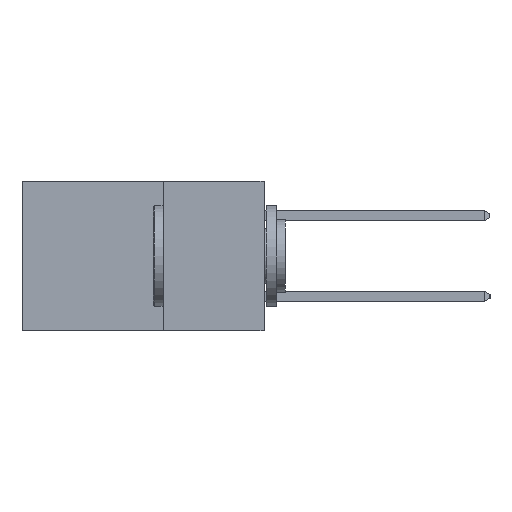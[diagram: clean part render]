
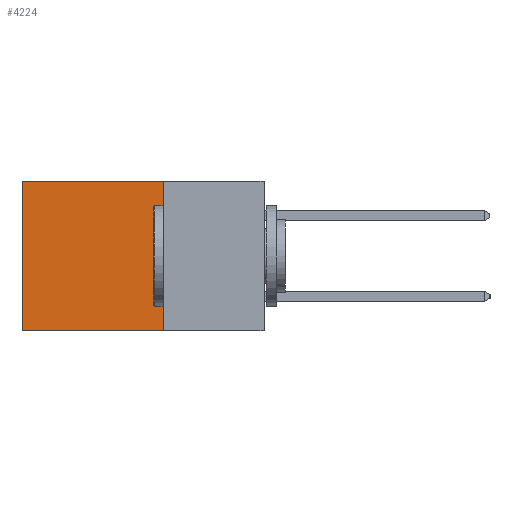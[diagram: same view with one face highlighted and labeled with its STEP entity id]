
A CAD part, left-side view. The second image highlights one B-rep face of the part: STEP entity #4224.
In plain terms, the highlighted planar face has unit normal (-1, 0, 0).
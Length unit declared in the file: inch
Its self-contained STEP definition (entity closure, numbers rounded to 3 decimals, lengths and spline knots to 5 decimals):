
#299 = EDGE_CURVE ( 'NONE', #1886, #1683, #7011, .T. ) ;
#606 = CARTESIAN_POINT ( 'NONE',  ( 0.2615, 0.6, -0.37 ) ) ;
#1332 = ORIENTED_EDGE ( 'NONE', *, *, #299, .T. ) ;
#1342 = EDGE_CURVE ( 'NONE', #7240, #1683, #8126, .T. ) ;
#1373 = EDGE_CURVE ( 'NONE', #3630, #1886, #9431, .T. ) ;
#1683 = VERTEX_POINT ( 'NONE', #4598 ) ;
#1873 = DIRECTION ( 'NONE',  ( 0., 0., -1. ) ) ;
#1886 = VERTEX_POINT ( 'NONE', #8300 ) ;
#2322 = EDGE_CURVE ( 'NONE', #3630, #7240, #6448, .T. ) ;
#2398 = VECTOR ( 'NONE', #4538, 39.37008 ) ;
#3630 = VERTEX_POINT ( 'NONE', #8421 ) ;
#3637 = PLANE ( 'NONE',  #4734 ) ;
#3781 = CARTESIAN_POINT ( 'NONE',  ( 0.2615, 0.25, -0.37 ) ) ;
#4224 = ADVANCED_FACE ( 'NONE', ( #4765 ), #3637, .F. ) ;
#4274 = VECTOR ( 'NONE', #9451, 39.37008 ) ;
#4538 = DIRECTION ( 'NONE',  ( 0., 0., -1. ) ) ;
#4598 = CARTESIAN_POINT ( 'NONE',  ( 0.2615, 0.6, -0.37 ) ) ;
#4734 = AXIS2_PLACEMENT_3D ( 'NONE', #6534, #9142, #1873 ) ;
#4765 = FACE_OUTER_BOUND ( 'NONE', #4913, .T. ) ;
#4913 = EDGE_LOOP ( 'NONE', ( #1332, #9201, #7678, #7879 ) ) ;
#5254 = DIRECTION ( 'NONE',  ( 0., 0., -1. ) ) ;
#5960 = VECTOR ( 'NONE', #7047, 39.37008 ) ;
#6133 = CARTESIAN_POINT ( 'NONE',  ( 0.2615, 0.25, 0. ) ) ;
#6418 = CARTESIAN_POINT ( 'NONE',  ( 0.2615, 0.25, -0.37 ) ) ;
#6448 = LINE ( 'NONE', #3781, #2398 ) ;
#6534 = CARTESIAN_POINT ( 'NONE',  ( 0.2615, 0.25, -0.37 ) ) ;
#7011 = LINE ( 'NONE', #606, #7216 ) ;
#7047 = DIRECTION ( 'NONE',  ( 0., 1., 0. ) ) ;
#7216 = VECTOR ( 'NONE', #5254, 39.37008 ) ;
#7240 = VERTEX_POINT ( 'NONE', #9492 ) ;
#7678 = ORIENTED_EDGE ( 'NONE', *, *, #2322, .F. ) ;
#7879 = ORIENTED_EDGE ( 'NONE', *, *, #1373, .T. ) ;
#8126 = LINE ( 'NONE', #6418, #4274 ) ;
#8300 = CARTESIAN_POINT ( 'NONE',  ( 0.2615, 0.6, 0. ) ) ;
#8421 = CARTESIAN_POINT ( 'NONE',  ( 0.2615, 0.25, 0. ) ) ;
#9142 = DIRECTION ( 'NONE',  ( 1., 0., 0. ) ) ;
#9201 = ORIENTED_EDGE ( 'NONE', *, *, #1342, .F. ) ;
#9431 = LINE ( 'NONE', #6133, #5960 ) ;
#9451 = DIRECTION ( 'NONE',  ( 0., 1., 0. ) ) ;
#9492 = CARTESIAN_POINT ( 'NONE',  ( 0.2615, 0.25, -0.37 ) ) ;
